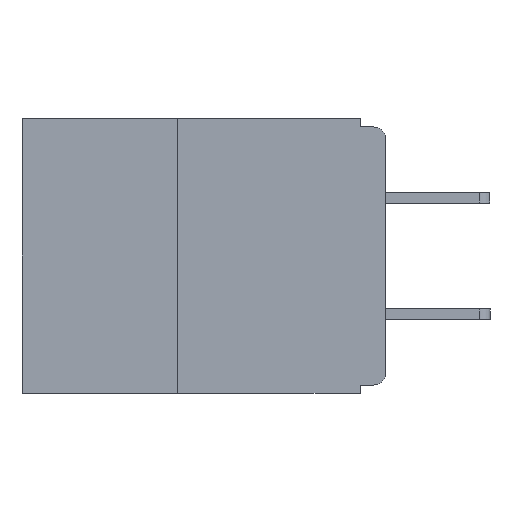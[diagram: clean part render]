
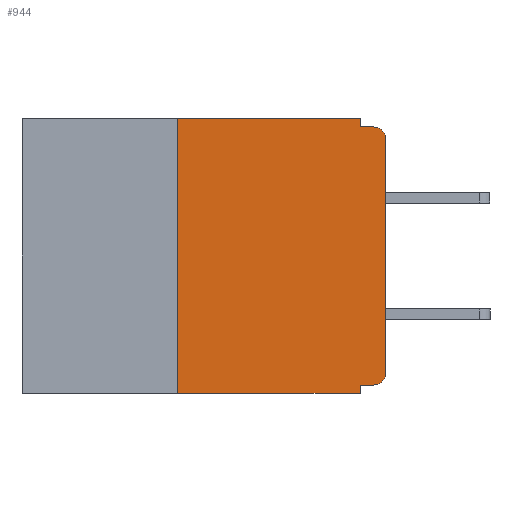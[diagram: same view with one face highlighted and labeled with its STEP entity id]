
A CAD part, left-side view. The second image highlights one B-rep face of the part: STEP entity #944.
In plain terms, the highlighted planar face has unit normal (-1, 0, 0).
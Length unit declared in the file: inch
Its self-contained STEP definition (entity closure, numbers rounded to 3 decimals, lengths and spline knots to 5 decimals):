
#810 = CARTESIAN_POINT ( 'NONE',  ( 0., 0.031, -0.33 ) ) ;
#907 = DIRECTION ( 'NONE',  ( 0., 0., -1. ) ) ;
#944 = ADVANCED_FACE ( 'NONE', ( #7214 ), #13514, .F. ) ;
#1145 = CARTESIAN_POINT ( 'NONE',  ( 0., 0.015, -0.025 ) ) ;
#1300 = LINE ( 'NONE', #21435, #10931 ) ;
#2077 = DIRECTION ( 'NONE',  ( 0., -1., 0. ) ) ;
#2533 = DIRECTION ( 'NONE',  ( 0., 0., 1. ) ) ;
#2591 = VERTEX_POINT ( 'NONE', #21785 ) ;
#2732 = EDGE_CURVE ( 'NONE', #19185, #4586, #16485, .T. ) ;
#2814 = CARTESIAN_POINT ( 'NONE',  ( 0., 0.25, -0.33 ) ) ;
#3029 = DIRECTION ( 'NONE',  ( 0., 0., -1. ) ) ;
#3437 = EDGE_LOOP ( 'NONE', ( #13137, #15505, #23991, #18706, #7963, #11917, #24223, #18089, #19514, #3706 ) ) ;
#3706 = ORIENTED_EDGE ( 'NONE', *, *, #21780, .T. ) ;
#3794 = DIRECTION ( 'NONE',  ( 0., 0., -1. ) ) ;
#3859 = EDGE_CURVE ( 'NONE', #23957, #14544, #20154, .T. ) ;
#3939 = DIRECTION ( 'NONE',  ( -1., 0., 0. ) ) ;
#4068 = AXIS2_PLACEMENT_3D ( 'NONE', #15490, #3939, #17372 ) ;
#4586 = VERTEX_POINT ( 'NONE', #16272 ) ;
#4712 = LINE ( 'NONE', #23151, #14422 ) ;
#5103 = EDGE_CURVE ( 'NONE', #2591, #24213, #17376, .T. ) ;
#6009 = DIRECTION ( 'NONE',  ( 0., 1., 0. ) ) ;
#6389 = LINE ( 'NONE', #11835, #16068 ) ;
#6397 = EDGE_CURVE ( 'NONE', #2591, #11497, #4712, .T. ) ;
#6869 = VERTEX_POINT ( 'NONE', #10910 ) ;
#7214 = FACE_OUTER_BOUND ( 'NONE', #3437, .T. ) ;
#7739 = EDGE_CURVE ( 'NONE', #13954, #11497, #16133, .T. ) ;
#7873 = CARTESIAN_POINT ( 'NONE',  ( 0., 0.031, 0. ) ) ;
#7963 = ORIENTED_EDGE ( 'NONE', *, *, #10011, .F. ) ;
#8450 = AXIS2_PLACEMENT_3D ( 'NONE', #1145, #14598, #3029 ) ;
#8564 = LINE ( 'NONE', #13607, #13669 ) ;
#9223 = EDGE_CURVE ( 'NONE', #14544, #22116, #8564, .T. ) ;
#10011 = EDGE_CURVE ( 'NONE', #24213, #23957, #1300, .T. ) ;
#10910 = CARTESIAN_POINT ( 'NONE',  ( 0., 0.015, -0.32 ) ) ;
#10931 = VECTOR ( 'NONE', #23205, 39.37008 ) ;
#11048 = VECTOR ( 'NONE', #907, 39.37008 ) ;
#11440 = VECTOR ( 'NONE', #24218, 39.37008 ) ;
#11497 = VERTEX_POINT ( 'NONE', #21187 ) ;
#11835 = CARTESIAN_POINT ( 'NONE',  ( 0., 0., -0.32 ) ) ;
#11917 = ORIENTED_EDGE ( 'NONE', *, *, #5103, .F. ) ;
#12002 = CARTESIAN_POINT ( 'NONE',  ( 0., 0.031, 0. ) ) ;
#12378 = CARTESIAN_POINT ( 'NONE',  ( 0., 0.031, -0.01 ) ) ;
#12497 = CARTESIAN_POINT ( 'NONE',  ( 0., 0., 0. ) ) ;
#12553 = DIRECTION ( 'NONE',  ( 0., 0., -1. ) ) ;
#12605 = DIRECTION ( 'NONE',  ( 1., 0., 0. ) ) ;
#13137 = ORIENTED_EDGE ( 'NONE', *, *, #2732, .T. ) ;
#13514 = PLANE ( 'NONE',  #18005 ) ;
#13544 = VECTOR ( 'NONE', #2533, 39.37008 ) ;
#13607 = CARTESIAN_POINT ( 'NONE',  ( 0., 0., -0.01 ) ) ;
#13669 = VECTOR ( 'NONE', #2077, 39.37008 ) ;
#13682 = CARTESIAN_POINT ( 'NONE',  ( 0., 0.437, 0. ) ) ;
#13880 = CIRCLE ( 'NONE', #8450, 0.015 ) ;
#13954 = VERTEX_POINT ( 'NONE', #17645 ) ;
#14002 = CARTESIAN_POINT ( 'NONE',  ( 0., 0., -0.305 ) ) ;
#14422 = VECTOR ( 'NONE', #23181, 39.37008 ) ;
#14544 = VERTEX_POINT ( 'NONE', #12378 ) ;
#14598 = DIRECTION ( 'NONE',  ( -1., 0., 0. ) ) ;
#14658 = CIRCLE ( 'NONE', #4068, 0.015 ) ;
#14755 = CARTESIAN_POINT ( 'NONE',  ( 0., 0.25, 0. ) ) ;
#15247 = VECTOR ( 'NONE', #3794, 39.37008 ) ;
#15490 = CARTESIAN_POINT ( 'NONE',  ( 0., 0.015, -0.305 ) ) ;
#15505 = ORIENTED_EDGE ( 'NONE', *, *, #19336, .T. ) ;
#15630 = EDGE_CURVE ( 'NONE', #6869, #13954, #6389, .T. ) ;
#16068 = VECTOR ( 'NONE', #6009, 39.37008 ) ;
#16133 = LINE ( 'NONE', #810, #11048 ) ;
#16272 = CARTESIAN_POINT ( 'NONE',  ( 0., 0., -0.025 ) ) ;
#16485 = LINE ( 'NONE', #12497, #11440 ) ;
#17372 = DIRECTION ( 'NONE',  ( 0., 0., -1. ) ) ;
#17376 = LINE ( 'NONE', #2814, #13544 ) ;
#17645 = CARTESIAN_POINT ( 'NONE',  ( 0., 0.031, -0.32 ) ) ;
#18005 = AXIS2_PLACEMENT_3D ( 'NONE', #13682, #12605, #12553 ) ;
#18089 = ORIENTED_EDGE ( 'NONE', *, *, #7739, .F. ) ;
#18706 = ORIENTED_EDGE ( 'NONE', *, *, #3859, .F. ) ;
#19185 = VERTEX_POINT ( 'NONE', #14002 ) ;
#19336 = EDGE_CURVE ( 'NONE', #4586, #22116, #13880, .T. ) ;
#19514 = ORIENTED_EDGE ( 'NONE', *, *, #15630, .F. ) ;
#20152 = CARTESIAN_POINT ( 'NONE',  ( 0., 0.015, -0.01 ) ) ;
#20154 = LINE ( 'NONE', #7873, #15247 ) ;
#21187 = CARTESIAN_POINT ( 'NONE',  ( 0., 0.031, -0.33 ) ) ;
#21435 = CARTESIAN_POINT ( 'NONE',  ( 0., 0.437, 0. ) ) ;
#21780 = EDGE_CURVE ( 'NONE', #6869, #19185, #14658, .T. ) ;
#21785 = CARTESIAN_POINT ( 'NONE',  ( 0., 0.25, -0.33 ) ) ;
#22116 = VERTEX_POINT ( 'NONE', #20152 ) ;
#23151 = CARTESIAN_POINT ( 'NONE',  ( 0., 0.437, -0.33 ) ) ;
#23181 = DIRECTION ( 'NONE',  ( 0., -1., 0. ) ) ;
#23205 = DIRECTION ( 'NONE',  ( 0., -1., 0. ) ) ;
#23957 = VERTEX_POINT ( 'NONE', #12002 ) ;
#23991 = ORIENTED_EDGE ( 'NONE', *, *, #9223, .F. ) ;
#24213 = VERTEX_POINT ( 'NONE', #14755 ) ;
#24218 = DIRECTION ( 'NONE',  ( 0., 0., 1. ) ) ;
#24223 = ORIENTED_EDGE ( 'NONE', *, *, #6397, .T. ) ;
